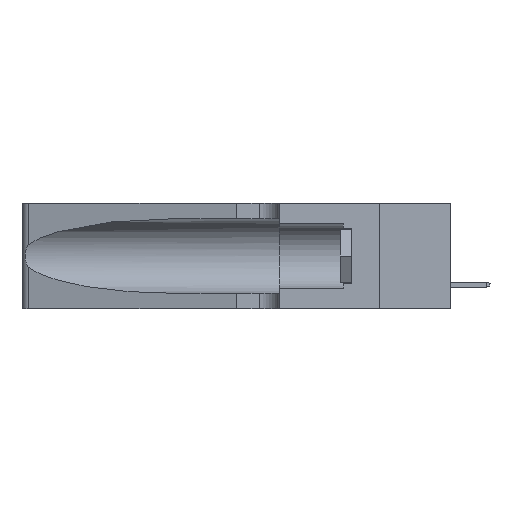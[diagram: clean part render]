
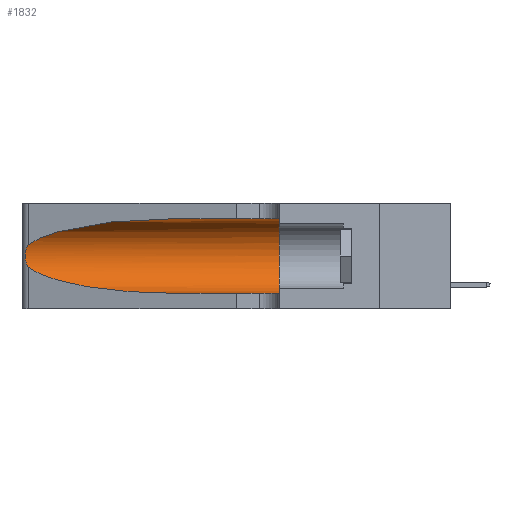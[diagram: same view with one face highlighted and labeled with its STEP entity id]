
A CAD part, left-side view. The second image highlights one B-rep face of the part: STEP entity #1832.
In plain terms, the highlighted cylindrical face has radius 3.308 mm (diameter 6.617 mm), a partial arc.
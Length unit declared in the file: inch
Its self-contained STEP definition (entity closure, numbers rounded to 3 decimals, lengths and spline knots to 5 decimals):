
#260 = CARTESIAN_POINT ( 'NONE',  ( 0.1305, 0.72297, 0.05475 ) ) ;
#410 = DIRECTION ( 'NONE',  ( 0., 0., 1. ) ) ;
#813 = CARTESIAN_POINT ( 'NONE',  ( 0.25487, 1.22718, 0.14631 ) ) ;
#960 = CARTESIAN_POINT ( 'NONE',  ( 0.26075, 1.23896, 0.19203 ) ) ;
#1074 = DIRECTION ( 'NONE',  ( 0., -1., 0. ) ) ;
#1405 = CARTESIAN_POINT ( 'NONE',  ( 0.26075, 1.23896, 0.178 ) ) ;
#1832 = ADVANCED_FACE ( 'NONE', ( #6016 ), #24124, .F. ) ;
#1926 = DIRECTION ( 'NONE',  ( 0., -1., 0. ) ) ;
#2887 = CARTESIAN_POINT ( 'NONE',  ( 0.1305, 0.72297, 0.05475 ) ) ;
#3206 = CARTESIAN_POINT ( 'NONE',  ( 0.25639, 1.23184, 0.21858 ) ) ;
#3232 = CARTESIAN_POINT ( 'NONE',  ( 0.1305, 0.72297, 0.31525 ) ) ;
#3286 = CARTESIAN_POINT ( 'NONE',  ( 0.2373, 1.15595, 0.28018 ) ) ;
#3459 = DIRECTION ( 'NONE',  ( 0., -1., 0. ) ) ;
#3481 = CARTESIAN_POINT ( 'NONE',  ( 0.25789, 1.23486, 0.15765 ) ) ;
#5397 = CARTESIAN_POINT ( 'NONE',  ( 0.18966, 0.96281, 0.31525 ) ) ;
#5876 = VERTEX_POINT ( 'NONE', #260 ) ;
#5919 = B_SPLINE_CURVE_WITH_KNOTS ( 'NONE', 3,
 ( #28467, #28329, #3206, #17288, #15010, #23997, #960, #1405, #10107, #21603, #3481, #14432, #28183, #813 ),
 .UNSPECIFIED., .F., .F.,
 ( 4, 2, 2, 2, 2, 2, 4 ),
 ( 0., 0.00027, 0.00053, 0.00107, 0.0016, 0.00187, 0.00214 ),
 .UNSPECIFIED. ) ;
#6016 = FACE_OUTER_BOUND ( 'NONE', #29155, .T. ) ;
#6428 = VERTEX_POINT ( 'NONE', #13189 ) ;
#6969 = ORIENTED_EDGE ( 'NONE', *, *, #13691, .T. ) ;
#7512 = CARTESIAN_POINT ( 'NONE',  ( 0.25487, 1.22718, 0.22369 ) ) ;
#7676 = EDGE_CURVE ( 'NONE', #9861, #11021, #25949, .T. ) ;
#8147 = VECTOR ( 'NONE', #1926, 39.37008 ) ;
#8671 = ORIENTED_EDGE ( 'NONE', *, *, #28842, .T. ) ;
#9616 = EDGE_CURVE ( 'NONE', #6428, #25495, #23681, .T. ) ;
#9861 = VERTEX_POINT ( 'NONE', #3232 ) ;
#10107 = CARTESIAN_POINT ( 'NONE',  ( 0.26017, 1.23833, 0.17102 ) ) ;
#11021 = VERTEX_POINT ( 'NONE', #24960 ) ;
#12472 = CARTESIAN_POINT ( 'NONE',  ( 0.1305, 1.61858, 0.185 ) ) ;
#12613 = DIRECTION ( 'NONE',  ( 0., 0., -1. ) ) ;
#13189 = CARTESIAN_POINT ( 'NONE',  ( 0.1305, 0.35, 0.31525 ) ) ;
#13327 = CARTESIAN_POINT ( 'NONE',  ( 0.1305, 0.35, 0.05475 ) ) ;
#13647 = AXIS2_PLACEMENT_3D ( 'NONE', #27622, #24809, #410 ) ;
#13691 = EDGE_CURVE ( 'NONE', #18010, #5876, #24025, .T. ) ;
#14432 = CARTESIAN_POINT ( 'NONE',  ( 0.25639, 1.23186, 0.15144 ) ) ;
#14911 = EDGE_CURVE ( 'NONE', #5876, #25495, #29258, .T. ) ;
#15010 = CARTESIAN_POINT ( 'NONE',  ( 0.25854, 1.2359, 0.20912 ) ) ;
#15978 = EDGE_CURVE ( 'NONE', #9861, #6428, #29280, .T. ) ;
#16076 = ORIENTED_EDGE ( 'NONE', *, *, #9616, .F. ) ;
#17288 = CARTESIAN_POINT ( 'NONE',  ( 0.25787, 1.23484, 0.2124 ) ) ;
#18010 = VERTEX_POINT ( 'NONE', #24745 ) ;
#18116 = VECTOR ( 'NONE', #1074, 39.37008 ) ;
#20997 = CARTESIAN_POINT ( 'NONE',  ( 0.25487, 1.22718, 0.14631 ) ) ;
#21406 = CARTESIAN_POINT ( 'NONE',  ( 0.1305, 0.72297, 0.31525 ) ) ;
#21603 = CARTESIAN_POINT ( 'NONE',  ( 0.25856, 1.23593, 0.16098 ) ) ;
#22567 = CARTESIAN_POINT ( 'NONE',  ( 0.1305, 1.61858, 0.31525 ) ) ;
#23389 = CARTESIAN_POINT ( 'NONE',  ( 0.18966, 0.96281, 0.05475 ) ) ;
#23410 = ORIENTED_EDGE ( 'NONE', *, *, #7676, .T. ) ;
#23681 = CIRCLE ( 'NONE', #13647, 0.13025 ) ;
#23997 = CARTESIAN_POINT ( 'NONE',  ( 0.26018, 1.23835, 0.19895 ) ) ;
#24025 =( BOUNDED_CURVE ( )  B_SPLINE_CURVE ( 3, ( #20997, #27716, #23389, #2887 ),
 .UNSPECIFIED., .F., .T. ) 
 B_SPLINE_CURVE_WITH_KNOTS ( ( 4, 4 ),
 ( 3.44316, 4.71239 ),
 .UNSPECIFIED. ) 
 CURVE ( )  GEOMETRIC_REPRESENTATION_ITEM ( )  RATIONAL_B_SPLINE_CURVE ( ( 1., 0.87, 0.87, 1. ) ) 
 REPRESENTATION_ITEM ( '' )  );
#24124 = CYLINDRICAL_SURFACE ( 'NONE', #24168, 0.13025 ) ;
#24168 = AXIS2_PLACEMENT_3D ( 'NONE', #12472, #3459, #12613 ) ;
#24745 = CARTESIAN_POINT ( 'NONE',  ( 0.25487, 1.22718, 0.14631 ) ) ;
#24809 = DIRECTION ( 'NONE',  ( 0., 1., 0. ) ) ;
#24960 = CARTESIAN_POINT ( 'NONE',  ( 0.25487, 1.22718, 0.22369 ) ) ;
#25488 = CARTESIAN_POINT ( 'NONE',  ( 0.1305, 1.61858, 0.05475 ) ) ;
#25495 = VERTEX_POINT ( 'NONE', #13327 ) ;
#25809 = ORIENTED_EDGE ( 'NONE', *, *, #14911, .T. ) ;
#25949 =( BOUNDED_CURVE ( )  B_SPLINE_CURVE ( 3, ( #21406, #5397, #3286, #7512 ),
 .UNSPECIFIED., .F., .T. ) 
 B_SPLINE_CURVE_WITH_KNOTS ( ( 4, 4 ),
 ( 1.5708, 2.84003 ),
 .UNSPECIFIED. ) 
 CURVE ( )  GEOMETRIC_REPRESENTATION_ITEM ( )  RATIONAL_B_SPLINE_CURVE ( ( 1., 0.87, 0.87, 1. ) ) 
 REPRESENTATION_ITEM ( '' )  );
#27622 = CARTESIAN_POINT ( 'NONE',  ( 0.1305, 0.35, 0.185 ) ) ;
#27716 = CARTESIAN_POINT ( 'NONE',  ( 0.2373, 1.15595, 0.08982 ) ) ;
#27746 = ORIENTED_EDGE ( 'NONE', *, *, #15978, .F. ) ;
#28183 = CARTESIAN_POINT ( 'NONE',  ( 0.25555, 1.22993, 0.14849 ) ) ;
#28329 = CARTESIAN_POINT ( 'NONE',  ( 0.25555, 1.22994, 0.2215 ) ) ;
#28467 = CARTESIAN_POINT ( 'NONE',  ( 0.25487, 1.22718, 0.22369 ) ) ;
#28842 = EDGE_CURVE ( 'NONE', #11021, #18010, #5919, .T. ) ;
#29155 = EDGE_LOOP ( 'NONE', ( #23410, #8671, #6969, #25809, #16076, #27746 ) ) ;
#29258 = LINE ( 'NONE', #25488, #18116 ) ;
#29280 = LINE ( 'NONE', #22567, #8147 ) ;
